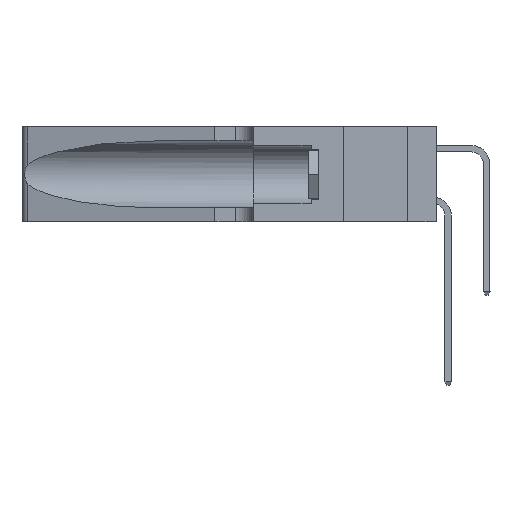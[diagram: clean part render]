
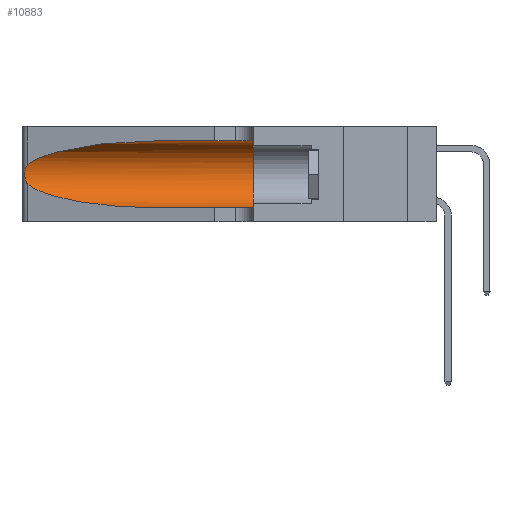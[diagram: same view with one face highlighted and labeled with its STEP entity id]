
A CAD part, left-side view. The second image highlights one B-rep face of the part: STEP entity #10883.
In plain terms, the highlighted cylindrical face has radius 3.308 mm (diameter 6.617 mm), a partial arc.
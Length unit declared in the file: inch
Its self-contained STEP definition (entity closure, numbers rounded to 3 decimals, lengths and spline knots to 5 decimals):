
#254 = VECTOR ( 'NONE', #18643, 39.37008 ) ;
#2035 = CARTESIAN_POINT ( 'NONE',  ( 0.18966, 0.96281, 0.31525 ) ) ;
#2060 = ORIENTED_EDGE ( 'NONE', *, *, #16549, .T. ) ;
#2287 = EDGE_LOOP ( 'NONE', ( #2060, #31730, #10874, #21466, #32656, #19254 ) ) ;
#2676 = VECTOR ( 'NONE', #30156, 39.37008 ) ;
#3406 = CARTESIAN_POINT ( 'NONE',  ( 0.1305, 1.61858, 0.31525 ) ) ;
#3740 = VERTEX_POINT ( 'NONE', #14489 ) ;
#4306 = VERTEX_POINT ( 'NONE', #5417 ) ;
#4463 = CARTESIAN_POINT ( 'NONE',  ( 0.25856, 1.23593, 0.16098 ) ) ;
#5185 =( BOUNDED_CURVE ( )  B_SPLINE_CURVE ( 3, ( #16946, #7794, #32213, #13989 ),
 .UNSPECIFIED., .F., .T. ) 
 B_SPLINE_CURVE_WITH_KNOTS ( ( 4, 4 ),
 ( 3.44316, 4.71239 ),
 .UNSPECIFIED. ) 
 CURVE ( )  GEOMETRIC_REPRESENTATION_ITEM ( )  RATIONAL_B_SPLINE_CURVE ( ( 1., 0.87, 0.87, 1. ) ) 
 REPRESENTATION_ITEM ( '' )  );
#5417 = CARTESIAN_POINT ( 'NONE',  ( 0.1305, 0.35, 0.31525 ) ) ;
#5492 = CARTESIAN_POINT ( 'NONE',  ( 0.1305, 1.61858, 0.05475 ) ) ;
#5523 = AXIS2_PLACEMENT_3D ( 'NONE', #27844, #37215, #12466 ) ;
#7230 = CARTESIAN_POINT ( 'NONE',  ( 0.25854, 1.2359, 0.20912 ) ) ;
#7794 = CARTESIAN_POINT ( 'NONE',  ( 0.2373, 1.15595, 0.08982 ) ) ;
#10120 = DIRECTION ( 'NONE',  ( 0., 1., 0. ) ) ;
#10275 = AXIS2_PLACEMENT_3D ( 'NONE', #28342, #10120, #13221 ) ;
#10329 = B_SPLINE_CURVE_WITH_KNOTS ( 'NONE', 3,
 ( #16390, #10334, #22514, #25563, #7230, #34747, #16531, #19565, #10468, #4463, #26594, #20149, #23206, #39064 ),
 .UNSPECIFIED., .F., .F.,
 ( 4, 2, 2, 2, 2, 2, 4 ),
 ( 0., 0.00027, 0.00053, 0.00107, 0.0016, 0.00187, 0.00214 ),
 .UNSPECIFIED. ) ;
#10334 = CARTESIAN_POINT ( 'NONE',  ( 0.25555, 1.22994, 0.2215 ) ) ;
#10415 = CARTESIAN_POINT ( 'NONE',  ( 0.25487, 1.22718, 0.22369 ) ) ;
#10468 = CARTESIAN_POINT ( 'NONE',  ( 0.26017, 1.23833, 0.17102 ) ) ;
#10874 = ORIENTED_EDGE ( 'NONE', *, *, #27396, .T. ) ;
#10883 = ADVANCED_FACE ( 'NONE', ( #17583 ), #17080, .F. ) ;
#11787 = EDGE_CURVE ( 'NONE', #35455, #12570, #33197, .T. ) ;
#12466 = DIRECTION ( 'NONE',  ( 0., 0., -1. ) ) ;
#12570 = VERTEX_POINT ( 'NONE', #13700 ) ;
#13221 = DIRECTION ( 'NONE',  ( 0., 0., 1. ) ) ;
#13700 = CARTESIAN_POINT ( 'NONE',  ( 0.1305, 0.35, 0.05475 ) ) ;
#13794 = CARTESIAN_POINT ( 'NONE',  ( 0.25487, 1.22718, 0.22369 ) ) ;
#13937 = VERTEX_POINT ( 'NONE', #38901 ) ;
#13989 = CARTESIAN_POINT ( 'NONE',  ( 0.1305, 0.72297, 0.05475 ) ) ;
#14489 = CARTESIAN_POINT ( 'NONE',  ( 0.25487, 1.22718, 0.14631 ) ) ;
#14619 = EDGE_CURVE ( 'NONE', #4306, #12570, #37214, .T. ) ;
#15341 = EDGE_CURVE ( 'NONE', #34858, #3740, #10329, .T. ) ;
#16390 = CARTESIAN_POINT ( 'NONE',  ( 0.25487, 1.22718, 0.22369 ) ) ;
#16531 = CARTESIAN_POINT ( 'NONE',  ( 0.26075, 1.23896, 0.19203 ) ) ;
#16549 = EDGE_CURVE ( 'NONE', #13937, #34858, #35267, .T. ) ;
#16946 = CARTESIAN_POINT ( 'NONE',  ( 0.25487, 1.22718, 0.14631 ) ) ;
#17080 = CYLINDRICAL_SURFACE ( 'NONE', #5523, 0.13025 ) ;
#17583 = FACE_OUTER_BOUND ( 'NONE', #2287, .T. ) ;
#18643 = DIRECTION ( 'NONE',  ( 0., -1., 0. ) ) ;
#19116 = CARTESIAN_POINT ( 'NONE',  ( 0.1305, 0.72297, 0.05475 ) ) ;
#19254 = ORIENTED_EDGE ( 'NONE', *, *, #39054, .F. ) ;
#19565 = CARTESIAN_POINT ( 'NONE',  ( 0.26075, 1.23896, 0.178 ) ) ;
#20149 = CARTESIAN_POINT ( 'NONE',  ( 0.25639, 1.23186, 0.15144 ) ) ;
#20327 = CARTESIAN_POINT ( 'NONE',  ( 0.1305, 0.72297, 0.31525 ) ) ;
#21466 = ORIENTED_EDGE ( 'NONE', *, *, #11787, .T. ) ;
#22514 = CARTESIAN_POINT ( 'NONE',  ( 0.25639, 1.23184, 0.21858 ) ) ;
#23206 = CARTESIAN_POINT ( 'NONE',  ( 0.25555, 1.22993, 0.14849 ) ) ;
#25563 = CARTESIAN_POINT ( 'NONE',  ( 0.25787, 1.23484, 0.2124 ) ) ;
#26594 = CARTESIAN_POINT ( 'NONE',  ( 0.25789, 1.23486, 0.15765 ) ) ;
#27396 = EDGE_CURVE ( 'NONE', #3740, #35455, #5185, .T. ) ;
#27844 = CARTESIAN_POINT ( 'NONE',  ( 0.1305, 1.61858, 0.185 ) ) ;
#28342 = CARTESIAN_POINT ( 'NONE',  ( 0.1305, 0.35, 0.185 ) ) ;
#29341 = LINE ( 'NONE', #3406, #254 ) ;
#30156 = DIRECTION ( 'NONE',  ( 0., -1., 0. ) ) ;
#31730 = ORIENTED_EDGE ( 'NONE', *, *, #15341, .T. ) ;
#32213 = CARTESIAN_POINT ( 'NONE',  ( 0.18966, 0.96281, 0.05475 ) ) ;
#32656 = ORIENTED_EDGE ( 'NONE', *, *, #14619, .F. ) ;
#33197 = LINE ( 'NONE', #5492, #2676 ) ;
#34747 = CARTESIAN_POINT ( 'NONE',  ( 0.26018, 1.23835, 0.19895 ) ) ;
#34858 = VERTEX_POINT ( 'NONE', #10415 ) ;
#35122 = CARTESIAN_POINT ( 'NONE',  ( 0.2373, 1.15595, 0.28018 ) ) ;
#35267 =( BOUNDED_CURVE ( )  B_SPLINE_CURVE ( 3, ( #20327, #2035, #35122, #13794 ),
 .UNSPECIFIED., .F., .T. ) 
 B_SPLINE_CURVE_WITH_KNOTS ( ( 4, 4 ),
 ( 1.5708, 2.84003 ),
 .UNSPECIFIED. ) 
 CURVE ( )  GEOMETRIC_REPRESENTATION_ITEM ( )  RATIONAL_B_SPLINE_CURVE ( ( 1., 0.87, 0.87, 1. ) ) 
 REPRESENTATION_ITEM ( '' )  );
#35455 = VERTEX_POINT ( 'NONE', #19116 ) ;
#37214 = CIRCLE ( 'NONE', #10275, 0.13025 ) ;
#37215 = DIRECTION ( 'NONE',  ( 0., -1., 0. ) ) ;
#38901 = CARTESIAN_POINT ( 'NONE',  ( 0.1305, 0.72297, 0.31525 ) ) ;
#39054 = EDGE_CURVE ( 'NONE', #13937, #4306, #29341, .T. ) ;
#39064 = CARTESIAN_POINT ( 'NONE',  ( 0.25487, 1.22718, 0.14631 ) ) ;
